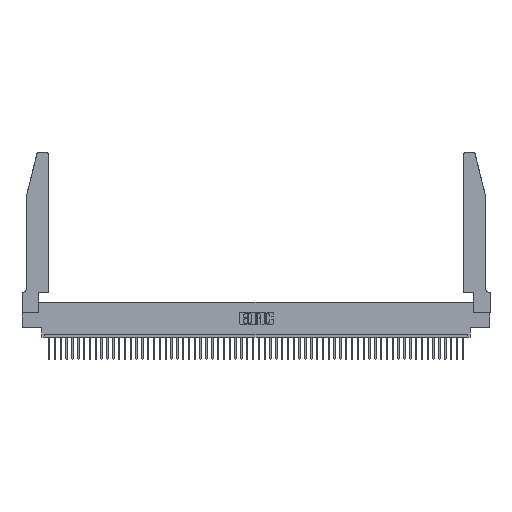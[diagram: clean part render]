
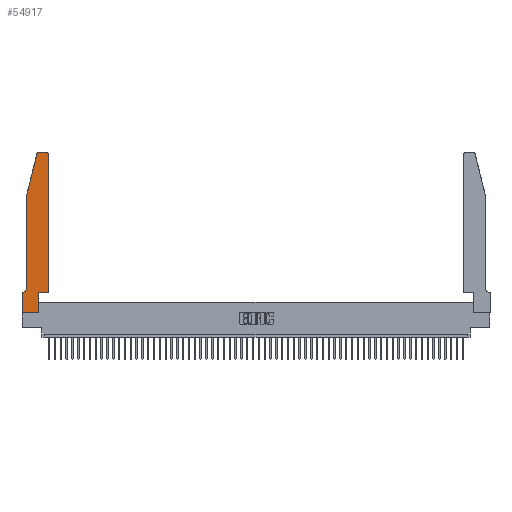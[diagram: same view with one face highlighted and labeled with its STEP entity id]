
A CAD part, top view. The second image highlights one B-rep face of the part: STEP entity #54917.
In plain terms, the highlighted planar face has unit normal (0, 0, 1).
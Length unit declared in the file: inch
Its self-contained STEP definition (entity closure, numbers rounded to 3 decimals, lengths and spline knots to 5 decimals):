
#680 = VECTOR ( 'NONE', #27841, 39.37008 ) ;
#1955 = CARTESIAN_POINT ( 'NONE',  ( 0.2865, 0.35, 0.37 ) ) ;
#1999 = VECTOR ( 'NONE', #29151, 39.37008 ) ;
#2984 = DIRECTION ( 'NONE',  ( 0., 0., 1. ) ) ;
#3941 = EDGE_CURVE ( 'NONE', #50906, #47272, #8524, .T. ) ;
#4598 = LINE ( 'NONE', #23303, #34540 ) ;
#4624 = DIRECTION ( 'NONE',  ( 0., -1., 0. ) ) ;
#5334 = AXIS2_PLACEMENT_3D ( 'NONE', #24977, #2984, #32769 ) ;
#5833 = CARTESIAN_POINT ( 'NONE',  ( 0.4505, 0.35, 0.37 ) ) ;
#5904 = ORIENTED_EDGE ( 'NONE', *, *, #46768, .T. ) ;
#6831 = CIRCLE ( 'NONE', #13441, 0.07 ) ;
#7426 = ORIENTED_EDGE ( 'NONE', *, *, #9223, .T. ) ;
#7442 = VERTEX_POINT ( 'NONE', #16343 ) ;
#7746 = CARTESIAN_POINT ( 'NONE',  ( 0.4205, 2.75, 0.37 ) ) ;
#8176 = LINE ( 'NONE', #33631, #26745 ) ;
#8355 = ORIENTED_EDGE ( 'NONE', *, *, #46889, .T. ) ;
#8524 = LINE ( 'NONE', #50379, #21191 ) ;
#8931 = AXIS2_PLACEMENT_3D ( 'NONE', #36909, #15810, #45444 ) ;
#9152 = VECTOR ( 'NONE', #29706, 39.37008 ) ;
#9223 = EDGE_CURVE ( 'NONE', #44734, #36824, #44949, .T. ) ;
#9842 = VERTEX_POINT ( 'NONE', #11996 ) ;
#10836 = FACE_OUTER_BOUND ( 'NONE', #32011, .T. ) ;
#11996 = CARTESIAN_POINT ( 'NONE',  ( 0.0755, 2., 0.37 ) ) ;
#12579 = EDGE_CURVE ( 'NONE', #22546, #24255, #52604, .T. ) ;
#13374 = LINE ( 'NONE', #33820, #1999 ) ;
#13441 = AXIS2_PLACEMENT_3D ( 'NONE', #24844, #39011, #17905 ) ;
#13508 = EDGE_CURVE ( 'NONE', #46938, #50906, #16123, .T. ) ;
#13529 = DIRECTION ( 'NONE',  ( 1., 0., 0. ) ) ;
#14670 = DIRECTION ( 'NONE',  ( -1., 0., 0. ) ) ;
#15036 = AXIS2_PLACEMENT_3D ( 'NONE', #16454, #20710, #13529 ) ;
#15113 = LINE ( 'NONE', #26515, #37661 ) ;
#15215 = LINE ( 'NONE', #28123, #9152 ) ;
#15810 = DIRECTION ( 'NONE',  ( 0., 0., 1. ) ) ;
#16123 = LINE ( 'NONE', #36540, #45217 ) ;
#16343 = CARTESIAN_POINT ( 'NONE',  ( 0.4505, 2.72, 0.37 ) ) ;
#16408 = DIRECTION ( 'NONE',  ( -1., 0., 0. ) ) ;
#16454 = CARTESIAN_POINT ( 'NONE',  ( 0.4205, 2.72, 0.37 ) ) ;
#17905 = DIRECTION ( 'NONE',  ( -1., 0., 0. ) ) ;
#20202 = EDGE_CURVE ( 'NONE', #24255, #7442, #4598, .T. ) ;
#20710 = DIRECTION ( 'NONE',  ( 0., 0., 1. ) ) ;
#21191 = VECTOR ( 'NONE', #4624, 39.37008 ) ;
#22546 = VERTEX_POINT ( 'NONE', #53168 ) ;
#23070 = ORIENTED_EDGE ( 'NONE', *, *, #38583, .T. ) ;
#23303 = CARTESIAN_POINT ( 'NONE',  ( 0.4505, 0.35, 0.37 ) ) ;
#24255 = VERTEX_POINT ( 'NONE', #40277 ) ;
#24844 = CARTESIAN_POINT ( 'NONE',  ( 0.0055, 0.42, 0.37 ) ) ;
#24977 = CARTESIAN_POINT ( 'NONE',  ( 0.284, 2.72, 0.37 ) ) ;
#25603 = ORIENTED_EDGE ( 'NONE', *, *, #42655, .T. ) ;
#26049 = VERTEX_POINT ( 'NONE', #7746 ) ;
#26506 = ORIENTED_EDGE ( 'NONE', *, *, #32960, .T. ) ;
#26515 = CARTESIAN_POINT ( 'NONE',  ( 0., 0., 0.37 ) ) ;
#26724 = VERTEX_POINT ( 'NONE', #33635 ) ;
#26745 = VECTOR ( 'NONE', #16408, 39.37008 ) ;
#27274 = EDGE_CURVE ( 'NONE', #47272, #37656, #15113, .T. ) ;
#27841 = DIRECTION ( 'NONE',  ( 1., 0., 0. ) ) ;
#27855 = DIRECTION ( 'NONE',  ( 0., 1., 0. ) ) ;
#28123 = CARTESIAN_POINT ( 'NONE',  ( 0.0755, 2., 0.37 ) ) ;
#28256 = ORIENTED_EDGE ( 'NONE', *, *, #13508, .T. ) ;
#29151 = DIRECTION ( 'NONE',  ( -0.239, -0.971, 0. ) ) ;
#29706 = DIRECTION ( 'NONE',  ( 0., -1., 0. ) ) ;
#30737 = DIRECTION ( 'NONE',  ( 1., 0., 0. ) ) ;
#32011 = EDGE_LOOP ( 'NONE', ( #8355, #7426, #23070, #26506, #48678, #28256, #49132, #52021, #5904, #47916, #40406, #25603 ) ) ;
#32267 = CARTESIAN_POINT ( 'NONE',  ( 0., 0., 0.37 ) ) ;
#32665 = PLANE ( 'NONE',  #8931 ) ;
#32769 = DIRECTION ( 'NONE',  ( 1., 0., 0. ) ) ;
#32960 = EDGE_CURVE ( 'NONE', #9842, #26724, #15215, .T. ) ;
#32983 = CARTESIAN_POINT ( 'NONE',  ( 0.2865, 0., 0.37 ) ) ;
#33631 = CARTESIAN_POINT ( 'NONE',  ( 0.2605, 2.75, 0.37 ) ) ;
#33635 = CARTESIAN_POINT ( 'NONE',  ( 0.0755, 0.42, 0.37 ) ) ;
#33653 = CARTESIAN_POINT ( 'NONE',  ( 0.25487, 2.72718, 0.37 ) ) ;
#33820 = CARTESIAN_POINT ( 'NONE',  ( 0.0755, 2., 0.37 ) ) ;
#34540 = VECTOR ( 'NONE', #43671, 39.37008 ) ;
#35880 = CARTESIAN_POINT ( 'NONE',  ( 0.284, 2.75, 0.37 ) ) ;
#36442 = CARTESIAN_POINT ( 'NONE',  ( 0., 0.35, 0.37 ) ) ;
#36540 = CARTESIAN_POINT ( 'NONE',  ( 0.0755, 0.35, 0.37 ) ) ;
#36617 = CIRCLE ( 'NONE', #15036, 0.03 ) ;
#36824 = VERTEX_POINT ( 'NONE', #33653 ) ;
#36909 = CARTESIAN_POINT ( 'NONE',  ( 0., 0.35, 0.37 ) ) ;
#37447 = VECTOR ( 'NONE', #27855, 39.37008 ) ;
#37545 = EDGE_CURVE ( 'NONE', #26724, #46938, #6831, .T. ) ;
#37656 = VERTEX_POINT ( 'NONE', #32983 ) ;
#37661 = VECTOR ( 'NONE', #30737, 39.37008 ) ;
#38583 = EDGE_CURVE ( 'NONE', #36824, #9842, #13374, .T. ) ;
#39011 = DIRECTION ( 'NONE',  ( 0., 0., -1. ) ) ;
#40277 = CARTESIAN_POINT ( 'NONE',  ( 0.4505, 0.35, 0.37 ) ) ;
#40406 = ORIENTED_EDGE ( 'NONE', *, *, #20202, .T. ) ;
#42655 = EDGE_CURVE ( 'NONE', #7442, #26049, #36617, .T. ) ;
#43671 = DIRECTION ( 'NONE',  ( 0., 1., 0. ) ) ;
#44734 = VERTEX_POINT ( 'NONE', #35880 ) ;
#44949 = CIRCLE ( 'NONE', #5334, 0.03 ) ;
#45217 = VECTOR ( 'NONE', #14670, 39.37008 ) ;
#45444 = DIRECTION ( 'NONE',  ( 1., 0., 0. ) ) ;
#46060 = LINE ( 'NONE', #1955, #37447 ) ;
#46768 = EDGE_CURVE ( 'NONE', #37656, #22546, #46060, .T. ) ;
#46889 = EDGE_CURVE ( 'NONE', #26049, #44734, #8176, .T. ) ;
#46938 = VERTEX_POINT ( 'NONE', #50075 ) ;
#47272 = VERTEX_POINT ( 'NONE', #32267 ) ;
#47916 = ORIENTED_EDGE ( 'NONE', *, *, #12579, .T. ) ;
#48678 = ORIENTED_EDGE ( 'NONE', *, *, #37545, .T. ) ;
#49132 = ORIENTED_EDGE ( 'NONE', *, *, #3941, .T. ) ;
#50075 = CARTESIAN_POINT ( 'NONE',  ( 0.0055, 0.35, 0.37 ) ) ;
#50379 = CARTESIAN_POINT ( 'NONE',  ( 0., 0., 0.37 ) ) ;
#50906 = VERTEX_POINT ( 'NONE', #36442 ) ;
#52021 = ORIENTED_EDGE ( 'NONE', *, *, #27274, .T. ) ;
#52604 = LINE ( 'NONE', #5833, #680 ) ;
#53168 = CARTESIAN_POINT ( 'NONE',  ( 0.2865, 0.35, 0.37 ) ) ;
#54917 = ADVANCED_FACE ( 'NONE', ( #10836 ), #32665, .T. ) ;
